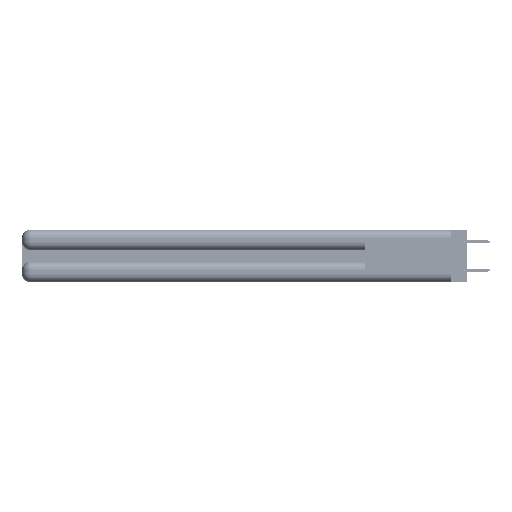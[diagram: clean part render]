
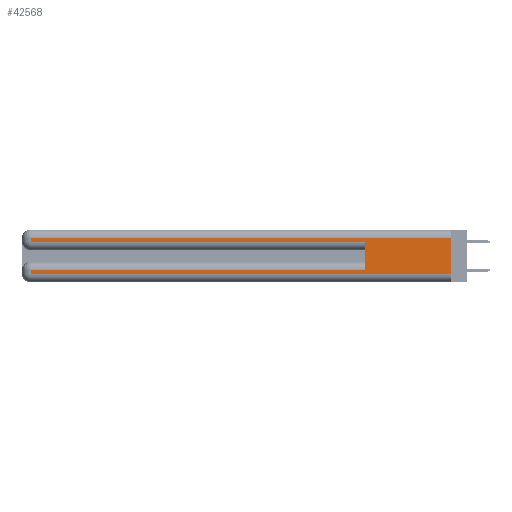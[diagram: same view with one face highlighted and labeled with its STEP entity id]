
A CAD part, left-side view. The second image highlights one B-rep face of the part: STEP entity #42568.
In plain terms, the highlighted planar face has unit normal (-1, 0, 0).
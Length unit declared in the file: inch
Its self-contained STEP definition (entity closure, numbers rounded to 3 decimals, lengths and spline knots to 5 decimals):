
#22 = LINE ( 'NONE', #34863, #20608 ) ;
#277 = VERTEX_POINT ( 'NONE', #11957 ) ;
#3097 = DIRECTION ( 'NONE',  ( 1., 0., 0. ) ) ;
#3237 = EDGE_CURVE ( 'NONE', #37850, #34582, #34061, .T. ) ;
#3513 = EDGE_CURVE ( 'NONE', #16000, #35115, #38537, .T. ) ;
#3585 = CARTESIAN_POINT ( 'NONE',  ( 0., 0., 0.085 ) ) ;
#3851 = ORIENTED_EDGE ( 'NONE', *, *, #33365, .F. ) ;
#4212 = CARTESIAN_POINT ( 'NONE',  ( 0., 0., 0.285 ) ) ;
#5461 = ORIENTED_EDGE ( 'NONE', *, *, #31718, .T. ) ;
#7757 = VECTOR ( 'NONE', #41634, 39.37008 ) ;
#8138 = EDGE_LOOP ( 'NONE', ( #24344, #5461, #37784, #32816, #3851, #40411, #50442, #14155 ) ) ;
#11194 = VERTEX_POINT ( 'NONE', #15696 ) ;
#11957 = CARTESIAN_POINT ( 'NONE',  ( 0., 0.6, 0.285 ) ) ;
#12749 = CARTESIAN_POINT ( 'NONE',  ( 0., 2.94, 0.37 ) ) ;
#12987 = DIRECTION ( 'NONE',  ( 0., 1., 0. ) ) ;
#13108 = DIRECTION ( 'NONE',  ( 0., 0., -1. ) ) ;
#14155 = ORIENTED_EDGE ( 'NONE', *, *, #3513, .T. ) ;
#14341 = VECTOR ( 'NONE', #12987, 39.37008 ) ;
#15696 = CARTESIAN_POINT ( 'NONE',  ( 0., 0., 0.31 ) ) ;
#16000 = VERTEX_POINT ( 'NONE', #44795 ) ;
#16247 = LINE ( 'NONE', #45840, #14341 ) ;
#16392 = CARTESIAN_POINT ( 'NONE',  ( 0., 2.94, 0.285 ) ) ;
#17270 = VECTOR ( 'NONE', #39041, 39.37008 ) ;
#20608 = VECTOR ( 'NONE', #51477, 39.37008 ) ;
#22780 = VECTOR ( 'NONE', #32994, 39.37008 ) ;
#23167 = CARTESIAN_POINT ( 'NONE',  ( 0., 2.94, 0.37 ) ) ;
#24272 = CARTESIAN_POINT ( 'NONE',  ( 0., 0.6, 0.085 ) ) ;
#24302 = CARTESIAN_POINT ( 'NONE',  ( 0., 0., 0.37 ) ) ;
#24344 = ORIENTED_EDGE ( 'NONE', *, *, #50532, .F. ) ;
#25714 = VECTOR ( 'NONE', #27661, 39.37008 ) ;
#26556 = LINE ( 'NONE', #12749, #7757 ) ;
#27661 = DIRECTION ( 'NONE',  ( 0., 0., -1. ) ) ;
#27728 = EDGE_CURVE ( 'NONE', #32529, #16000, #26556, .T. ) ;
#28428 = PLANE ( 'NONE',  #45205 ) ;
#29520 = CARTESIAN_POINT ( 'NONE',  ( 0., 0., 0.37 ) ) ;
#31718 = EDGE_CURVE ( 'NONE', #11194, #37850, #16247, .T. ) ;
#32529 = VERTEX_POINT ( 'NONE', #47214 ) ;
#32816 = ORIENTED_EDGE ( 'NONE', *, *, #49861, .T. ) ;
#32994 = DIRECTION ( 'NONE',  ( 0., -1., 0. ) ) ;
#33365 = EDGE_CURVE ( 'NONE', #36877, #277, #22, .T. ) ;
#34061 = LINE ( 'NONE', #23167, #25714 ) ;
#34582 = VERTEX_POINT ( 'NONE', #16392 ) ;
#34798 = FACE_OUTER_BOUND ( 'NONE', #8138, .T. ) ;
#34863 = CARTESIAN_POINT ( 'NONE',  ( 0., 0.6, 0.145 ) ) ;
#35115 = VERTEX_POINT ( 'NONE', #39648 ) ;
#36821 = VECTOR ( 'NONE', #13108, 39.37008 ) ;
#36877 = VERTEX_POINT ( 'NONE', #24272 ) ;
#36926 = EDGE_CURVE ( 'NONE', #36877, #32529, #50539, .T. ) ;
#37784 = ORIENTED_EDGE ( 'NONE', *, *, #3237, .T. ) ;
#37850 = VERTEX_POINT ( 'NONE', #47916 ) ;
#38537 = LINE ( 'NONE', #38850, #17270 ) ;
#38850 = CARTESIAN_POINT ( 'NONE',  ( 0., 0., 0.06 ) ) ;
#39041 = DIRECTION ( 'NONE',  ( 0., -1., 0. ) ) ;
#39648 = CARTESIAN_POINT ( 'NONE',  ( 0., 0., 0.06 ) ) ;
#40411 = ORIENTED_EDGE ( 'NONE', *, *, #36926, .T. ) ;
#40514 = DIRECTION ( 'NONE',  ( 0., 1., 0. ) ) ;
#40816 = LINE ( 'NONE', #4212, #22780 ) ;
#41634 = DIRECTION ( 'NONE',  ( 0., 0., -1. ) ) ;
#42568 = ADVANCED_FACE ( 'NONE', ( #34798 ), #28428, .F. ) ;
#44795 = CARTESIAN_POINT ( 'NONE',  ( 0., 2.94, 0.06 ) ) ;
#45205 = AXIS2_PLACEMENT_3D ( 'NONE', #24302, #3097, #52449 ) ;
#45840 = CARTESIAN_POINT ( 'NONE',  ( 0., 0., 0.31 ) ) ;
#46042 = VECTOR ( 'NONE', #40514, 39.37008 ) ;
#47214 = CARTESIAN_POINT ( 'NONE',  ( 0., 2.94, 0.085 ) ) ;
#47857 = LINE ( 'NONE', #29520, #36821 ) ;
#47916 = CARTESIAN_POINT ( 'NONE',  ( 0., 2.94, 0.31 ) ) ;
#49861 = EDGE_CURVE ( 'NONE', #34582, #277, #40816, .T. ) ;
#50442 = ORIENTED_EDGE ( 'NONE', *, *, #27728, .T. ) ;
#50532 = EDGE_CURVE ( 'NONE', #11194, #35115, #47857, .T. ) ;
#50539 = LINE ( 'NONE', #3585, #46042 ) ;
#51477 = DIRECTION ( 'NONE',  ( 0., 0., 1. ) ) ;
#52449 = DIRECTION ( 'NONE',  ( 0., 0., -1. ) ) ;
